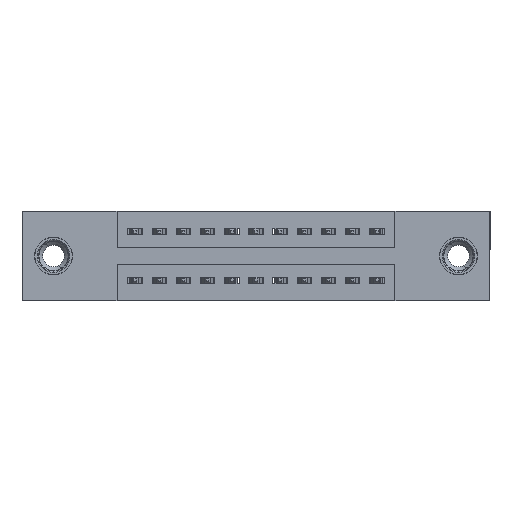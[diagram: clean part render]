
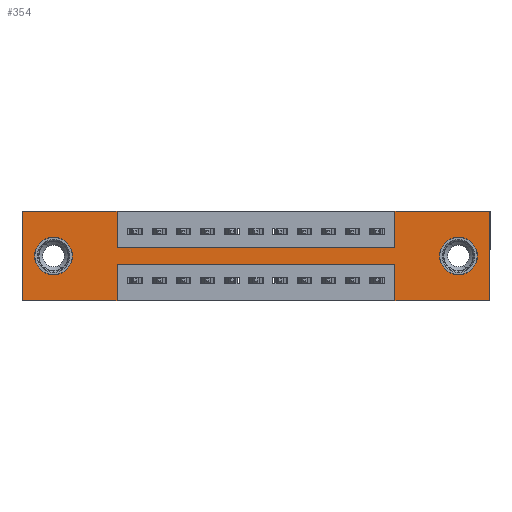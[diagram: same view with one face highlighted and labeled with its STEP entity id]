
A CAD part, front view. The second image highlights one B-rep face of the part: STEP entity #354.
In plain terms, the highlighted planar face has unit normal (0, -1, 0).
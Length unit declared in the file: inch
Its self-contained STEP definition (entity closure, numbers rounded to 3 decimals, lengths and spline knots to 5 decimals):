
#69 = VERTEX_POINT ( 'NONE', #8349 ) ;
#145 = VECTOR ( 'NONE', #17588, 39.37008 ) ;
#203 = VERTEX_POINT ( 'NONE', #9437 ) ;
#354 = ADVANCED_FACE ( 'NONE', ( #9955, #16852, #2938 ), #12643, .T. ) ;
#395 = ORIENTED_EDGE ( 'NONE', *, *, #9914, .T. ) ;
#413 = ORIENTED_EDGE ( 'NONE', *, *, #14755, .F. ) ;
#438 = CARTESIAN_POINT ( 'NONE',  ( 1.805, 0., -0.185 ) ) ;
#442 = EDGE_CURVE ( 'NONE', #3451, #17203, #12267, .T. ) ;
#676 = DIRECTION ( 'NONE',  ( 0., 0., 1. ) ) ;
#798 = CARTESIAN_POINT ( 'NONE',  ( 0.3925, 0., -0.15 ) ) ;
#835 = CARTESIAN_POINT ( 'NONE',  ( 0., 0., 0. ) ) ;
#1031 = VECTOR ( 'NONE', #15304, 39.37008 ) ;
#1044 = VERTEX_POINT ( 'NONE', #11347 ) ;
#1163 = VERTEX_POINT ( 'NONE', #10542 ) ;
#1394 = EDGE_CURVE ( 'NONE', #69, #1163, #6097, .T. ) ;
#1484 = LINE ( 'NONE', #3027, #1031 ) ;
#1542 = ORIENTED_EDGE ( 'NONE', *, *, #16751, .F. ) ;
#1619 = CARTESIAN_POINT ( 'NONE',  ( 0.13, 0., -0.185 ) ) ;
#1879 = DIRECTION ( 'NONE',  ( 0., 0., -1. ) ) ;
#1988 = DIRECTION ( 'NONE',  ( 0., 0., -1. ) ) ;
#2014 = DIRECTION ( 'NONE',  ( 0., -1., 0. ) ) ;
#2079 = VECTOR ( 'NONE', #3557, 39.37008 ) ;
#2221 = CARTESIAN_POINT ( 'NONE',  ( 0.13, 0., -0.185 ) ) ;
#2460 = CARTESIAN_POINT ( 'NONE',  ( 0.3925, 0., -0.37 ) ) ;
#2527 = CIRCLE ( 'NONE', #8853, 0.078 ) ;
#2550 = DIRECTION ( 'NONE',  ( -1., 0., 0. ) ) ;
#2656 = ORIENTED_EDGE ( 'NONE', *, *, #442, .T. ) ;
#2938 = FACE_OUTER_BOUND ( 'NONE', #16219, .T. ) ;
#3027 = CARTESIAN_POINT ( 'NONE',  ( 1.935, 0., 0. ) ) ;
#3083 = VECTOR ( 'NONE', #8196, 39.37008 ) ;
#3091 = DIRECTION ( 'NONE',  ( 0., 0., 1. ) ) ;
#3112 = CARTESIAN_POINT ( 'NONE',  ( 0.3925, 0., -0.22 ) ) ;
#3451 = VERTEX_POINT ( 'NONE', #10089 ) ;
#3487 = DIRECTION ( 'NONE',  ( 1., 0., 0. ) ) ;
#3557 = DIRECTION ( 'NONE',  ( 1., 0., 0. ) ) ;
#3867 = DIRECTION ( 'NONE',  ( -1., 0., 0. ) ) ;
#3876 = LINE ( 'NONE', #7673, #10810 ) ;
#3998 = VECTOR ( 'NONE', #3487, 39.37008 ) ;
#4033 = ORIENTED_EDGE ( 'NONE', *, *, #16816, .F. ) ;
#4293 = ORIENTED_EDGE ( 'NONE', *, *, #4868, .F. ) ;
#4295 = VERTEX_POINT ( 'NONE', #4897 ) ;
#4445 = LINE ( 'NONE', #9075, #3998 ) ;
#4516 = VERTEX_POINT ( 'NONE', #11145 ) ;
#4868 = EDGE_CURVE ( 'NONE', #9056, #16952, #13142, .T. ) ;
#4897 = CARTESIAN_POINT ( 'NONE',  ( 1.5425, 0., -0.37 ) ) ;
#4947 = EDGE_LOOP ( 'NONE', ( #11158, #395 ) ) ;
#4993 = CARTESIAN_POINT ( 'NONE',  ( 0., 0., 0. ) ) ;
#5121 = CIRCLE ( 'NONE', #15405, 0.078 ) ;
#5144 = ORIENTED_EDGE ( 'NONE', *, *, #5348, .T. ) ;
#5262 = DIRECTION ( 'NONE',  ( 0., 1., 0. ) ) ;
#5348 = EDGE_CURVE ( 'NONE', #17203, #3451, #2527, .T. ) ;
#5465 = VERTEX_POINT ( 'NONE', #16699 ) ;
#5721 = VERTEX_POINT ( 'NONE', #9349 ) ;
#5767 = CARTESIAN_POINT ( 'NONE',  ( 0.3925, 0., 0. ) ) ;
#5928 = EDGE_LOOP ( 'NONE', ( #5144, #2656 ) ) ;
#6097 = LINE ( 'NONE', #14747, #16272 ) ;
#6224 = EDGE_CURVE ( 'NONE', #4295, #5721, #3876, .T. ) ;
#6246 = EDGE_CURVE ( 'NONE', #13392, #5465, #14318, .T. ) ;
#6326 = EDGE_CURVE ( 'NONE', #1044, #4295, #6330, .T. ) ;
#6330 = LINE ( 'NONE', #7904, #16468 ) ;
#6338 = CARTESIAN_POINT ( 'NONE',  ( 0.3925, 0., -0.15 ) ) ;
#6449 = CARTESIAN_POINT ( 'NONE',  ( 0.13, 0., -0.107 ) ) ;
#6915 = LINE ( 'NONE', #17318, #14053 ) ;
#7180 = ORIENTED_EDGE ( 'NONE', *, *, #6246, .F. ) ;
#7195 = VERTEX_POINT ( 'NONE', #14155 ) ;
#7329 = LINE ( 'NONE', #5767, #145 ) ;
#7526 = CIRCLE ( 'NONE', #10474, 0.078 ) ;
#7673 = CARTESIAN_POINT ( 'NONE',  ( 1.5425, 0., -0.37 ) ) ;
#7815 = CARTESIAN_POINT ( 'NONE',  ( 1.5425, 0., 0. ) ) ;
#7904 = CARTESIAN_POINT ( 'NONE',  ( 0., 0., -0.37 ) ) ;
#8135 = AXIS2_PLACEMENT_3D ( 'NONE', #13294, #2014, #1988 ) ;
#8196 = DIRECTION ( 'NONE',  ( 0., 0., -1. ) ) ;
#8252 = ORIENTED_EDGE ( 'NONE', *, *, #6326, .F. ) ;
#8349 = CARTESIAN_POINT ( 'NONE',  ( 0.3925, 0., -0.37 ) ) ;
#8853 = AXIS2_PLACEMENT_3D ( 'NONE', #1619, #11413, #3091 ) ;
#8910 = EDGE_CURVE ( 'NONE', #16952, #13392, #7329, .T. ) ;
#9056 = VERTEX_POINT ( 'NONE', #11438 ) ;
#9075 = CARTESIAN_POINT ( 'NONE',  ( 0., 0., 0. ) ) ;
#9349 = CARTESIAN_POINT ( 'NONE',  ( 1.5425, 0., -0.22 ) ) ;
#9437 = CARTESIAN_POINT ( 'NONE',  ( 1.805, 0., -0.107 ) ) ;
#9732 = LINE ( 'NONE', #7815, #12887 ) ;
#9914 = EDGE_CURVE ( 'NONE', #15852, #203, #7526, .T. ) ;
#9955 = FACE_BOUND ( 'NONE', #4947, .T. ) ;
#10089 = CARTESIAN_POINT ( 'NONE',  ( 0.13, 0., -0.263 ) ) ;
#10299 = DIRECTION ( 'NONE',  ( 0., 1., 0. ) ) ;
#10474 = AXIS2_PLACEMENT_3D ( 'NONE', #438, #10299, #1879 ) ;
#10508 = LINE ( 'NONE', #2460, #3083 ) ;
#10542 = CARTESIAN_POINT ( 'NONE',  ( 0., 0., -0.37 ) ) ;
#10626 = DIRECTION ( 'NONE',  ( -1., 0., 0. ) ) ;
#10810 = VECTOR ( 'NONE', #15654, 39.37008 ) ;
#11145 = CARTESIAN_POINT ( 'NONE',  ( 1.5425, 0., 0. ) ) ;
#11158 = ORIENTED_EDGE ( 'NONE', *, *, #16488, .T. ) ;
#11347 = CARTESIAN_POINT ( 'NONE',  ( 1.935, 0., -0.37 ) ) ;
#11413 = DIRECTION ( 'NONE',  ( 0., 1., 0. ) ) ;
#11438 = CARTESIAN_POINT ( 'NONE',  ( 0., 0., 0. ) ) ;
#11731 = DIRECTION ( 'NONE',  ( 1., 0., 0. ) ) ;
#11985 = VECTOR ( 'NONE', #12024, 39.37008 ) ;
#12024 = DIRECTION ( 'NONE',  ( 0., 0., 1. ) ) ;
#12241 = ORIENTED_EDGE ( 'NONE', *, *, #15530, .F. ) ;
#12267 = CIRCLE ( 'NONE', #14376, 0.078 ) ;
#12406 = LINE ( 'NONE', #835, #11985 ) ;
#12643 = PLANE ( 'NONE',  #8135 ) ;
#12879 = ORIENTED_EDGE ( 'NONE', *, *, #16459, .F. ) ;
#12887 = VECTOR ( 'NONE', #676, 39.37008 ) ;
#13055 = ORIENTED_EDGE ( 'NONE', *, *, #1394, .F. ) ;
#13073 = ORIENTED_EDGE ( 'NONE', *, *, #13351, .F. ) ;
#13142 = LINE ( 'NONE', #4993, #2079 ) ;
#13294 = CARTESIAN_POINT ( 'NONE',  ( 0., 0., -0.37 ) ) ;
#13351 = EDGE_CURVE ( 'NONE', #5465, #4516, #9732, .T. ) ;
#13366 = CARTESIAN_POINT ( 'NONE',  ( 1.805, 0., -0.263 ) ) ;
#13392 = VERTEX_POINT ( 'NONE', #798 ) ;
#13406 = CARTESIAN_POINT ( 'NONE',  ( 1.805, 0., -0.185 ) ) ;
#14053 = VECTOR ( 'NONE', #2550, 39.37008 ) ;
#14155 = CARTESIAN_POINT ( 'NONE',  ( 1.935, 0., 0. ) ) ;
#14250 = DIRECTION ( 'NONE',  ( 0., 0., 1. ) ) ;
#14318 = LINE ( 'NONE', #6338, #17237 ) ;
#14376 = AXIS2_PLACEMENT_3D ( 'NONE', #2221, #14414, #14250 ) ;
#14414 = DIRECTION ( 'NONE',  ( 0., 1., 0. ) ) ;
#14698 = ORIENTED_EDGE ( 'NONE', *, *, #8910, .F. ) ;
#14719 = DIRECTION ( 'NONE',  ( 0., 0., -1. ) ) ;
#14747 = CARTESIAN_POINT ( 'NONE',  ( 0., 0., -0.37 ) ) ;
#14755 = EDGE_CURVE ( 'NONE', #5721, #17589, #6915, .T. ) ;
#15304 = DIRECTION ( 'NONE',  ( 0., 0., -1. ) ) ;
#15405 = AXIS2_PLACEMENT_3D ( 'NONE', #13406, #5262, #14719 ) ;
#15530 = EDGE_CURVE ( 'NONE', #7195, #1044, #1484, .T. ) ;
#15654 = DIRECTION ( 'NONE',  ( 0., 0., 1. ) ) ;
#15852 = VERTEX_POINT ( 'NONE', #13366 ) ;
#16219 = EDGE_LOOP ( 'NONE', ( #4033, #413, #17010, #8252, #12241, #1542, #13073, #7180, #14698, #4293, #12879, #13055 ) ) ;
#16272 = VECTOR ( 'NONE', #3867, 39.37008 ) ;
#16332 = CARTESIAN_POINT ( 'NONE',  ( 0.3925, 0., 0. ) ) ;
#16459 = EDGE_CURVE ( 'NONE', #1163, #9056, #12406, .T. ) ;
#16468 = VECTOR ( 'NONE', #10626, 39.37008 ) ;
#16488 = EDGE_CURVE ( 'NONE', #203, #15852, #5121, .T. ) ;
#16699 = CARTESIAN_POINT ( 'NONE',  ( 1.5425, 0., -0.15 ) ) ;
#16751 = EDGE_CURVE ( 'NONE', #4516, #7195, #4445, .T. ) ;
#16816 = EDGE_CURVE ( 'NONE', #17589, #69, #10508, .T. ) ;
#16852 = FACE_BOUND ( 'NONE', #5928, .T. ) ;
#16952 = VERTEX_POINT ( 'NONE', #16332 ) ;
#17010 = ORIENTED_EDGE ( 'NONE', *, *, #6224, .F. ) ;
#17203 = VERTEX_POINT ( 'NONE', #6449 ) ;
#17237 = VECTOR ( 'NONE', #11731, 39.37008 ) ;
#17318 = CARTESIAN_POINT ( 'NONE',  ( 0.3925, 0., -0.22 ) ) ;
#17588 = DIRECTION ( 'NONE',  ( 0., 0., -1. ) ) ;
#17589 = VERTEX_POINT ( 'NONE', #3112 ) ;
